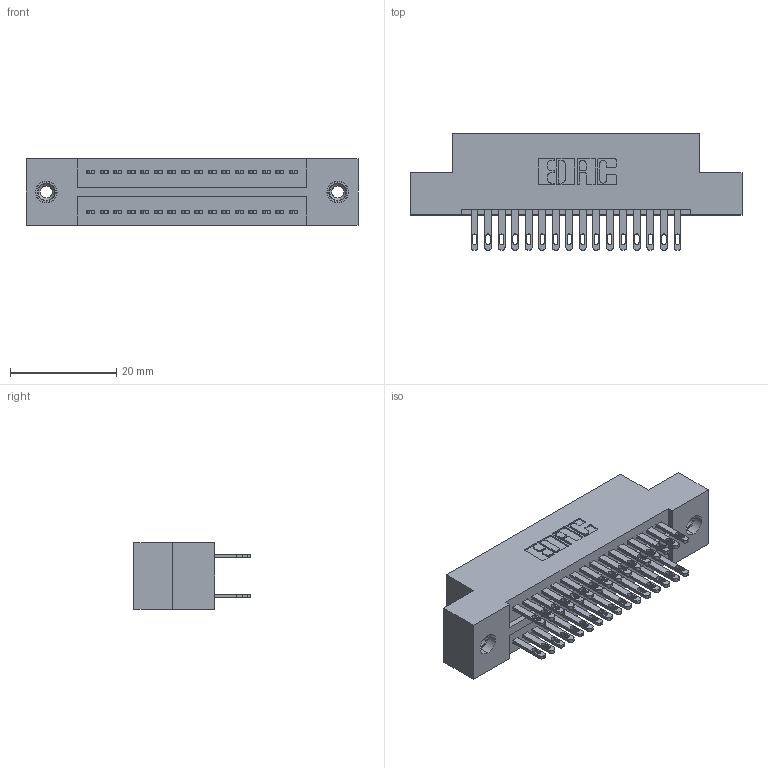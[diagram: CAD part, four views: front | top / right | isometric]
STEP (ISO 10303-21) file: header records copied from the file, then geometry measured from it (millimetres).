
FILE_DESCRIPTION (( 'STEP AP203' ), '1' );
FILE_NAME ('325-032-500-208.STEP', '2020-02-24T19:31:01', ( '' ), ( '' ), 'SwSTEP 2.0', 'SolidWorks 2016', '' );
FILE_SCHEMA (( 'CONFIG_CONTROL_DESIGN' ));
Length unit declared in the file: inch
Products named in the file (4): 325-292-001_325-293-100; 325-032-500-208; 345-250-001_345-250-003-102; 325 Part_TI
Assembly tree (35 placements, depth 2):
  325-032-500-208
    325 Part_TI
    325-292-001_325-293-100  x32
    345-250-001_345-250-003-102  x2
Bounding box: 62.36 x 21.84 x 12.45 mm (x, y, z)
Volume: 7908 mm3; surface area: 9303.3 mm2
Topology: 35 solids, 35 shells, 1710 faces, 5151 edges, 3426 vertices
Faces by surface type: plane 1062, cylinder 632, cone 12, torus 4
Entity records: 14772 total; most frequent: CARTESIAN_POINT 2461, ORIENTED_EDGE 2390, DIRECTION 2181, EDGE_CURVE 1195, VECTOR 1043, LINE 1043, VERTEX_POINT 792, AXIS2_PLACEMENT_3D 569
